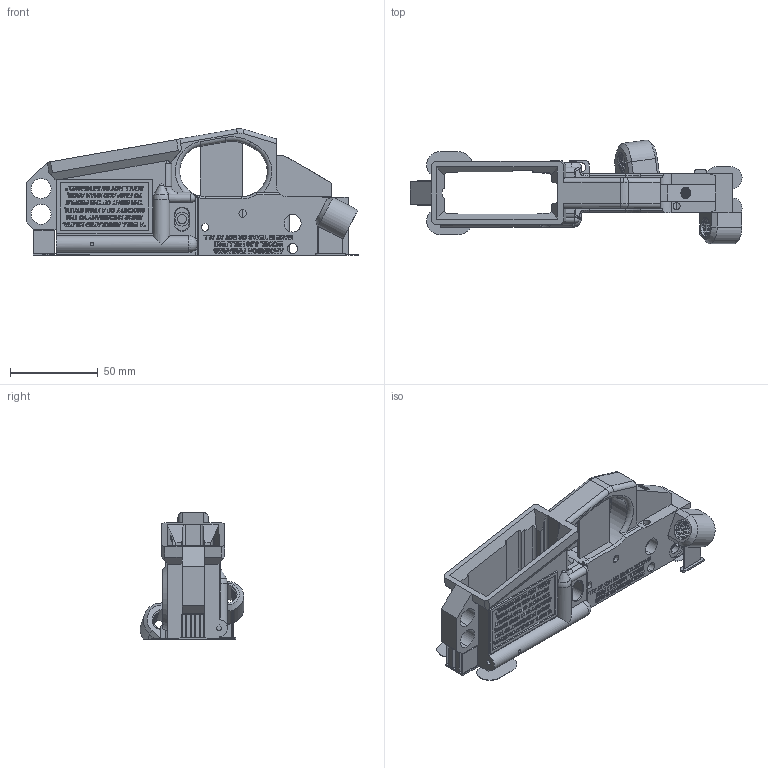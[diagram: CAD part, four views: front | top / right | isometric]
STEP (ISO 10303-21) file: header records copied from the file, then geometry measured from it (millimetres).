
FILE_DESCRIPTION (( 'STEP AP203' ), '1' );
FILE_NAME ('AF-HF-LR-PRT-008-STEP.STEP', '2020-11-04T14:30:41', ( '' ), ( '' ), 'SwSTEP 2.0', 'SolidWorks 2018', '' );
FILE_SCHEMA (( 'CONFIG_CONTROL_DESIGN' ));
Products named in the file (1): AF-HF-LR-PRT-008-STEP
Bounding box: 189.67 x 59.15 x 72.31 mm (x, y, z)
Volume: 102769 mm3; surface area: 75854.7 mm2
Topology: 5 solids, 5 shells, 3335 faces, 9128 edges, 6043 vertices
Faces by surface type: plane 2223, bspline 768, cylinder 299, torus 22, cone 19, sphere 4
Entity records: 186177 total; most frequent: CARTESIAN_POINT 107690, ORIENTED_EDGE 18244, DIRECTION 12811, EDGE_CURVE 9122, VECTOR 6681, LINE 6681, VERTEX_POINT 6042, EDGE_LOOP 3630
